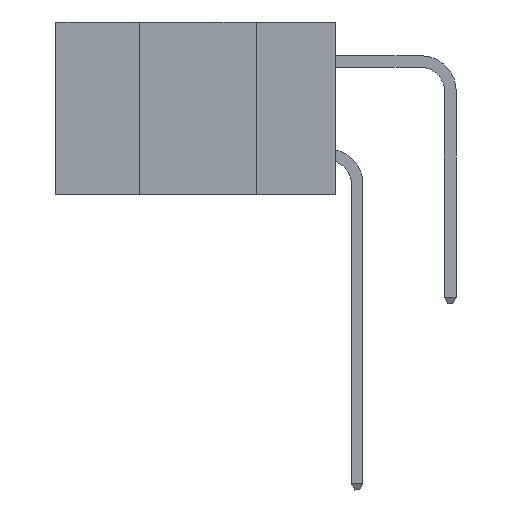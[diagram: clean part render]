
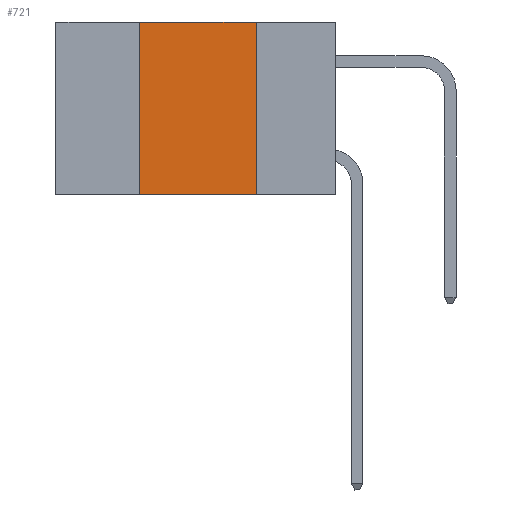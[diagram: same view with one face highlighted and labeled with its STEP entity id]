
A CAD part, left-side view. The second image highlights one B-rep face of the part: STEP entity #721.
In plain terms, the highlighted planar face has unit normal (-1, 0, 0).
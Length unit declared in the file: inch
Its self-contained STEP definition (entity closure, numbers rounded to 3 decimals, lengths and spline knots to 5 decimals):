
#721 = ADVANCED_FACE ( 'NONE', ( #14930 ), #4106, .F. ) ;
#874 = VECTOR ( 'NONE', #14177, 39.37008 ) ;
#1025 = CARTESIAN_POINT ( 'NONE',  ( 0., 0.17, -0.37 ) ) ;
#1962 = LINE ( 'NONE', #6880, #12260 ) ;
#2498 = CARTESIAN_POINT ( 'NONE',  ( 0., 0.17, 0. ) ) ;
#3488 = VERTEX_POINT ( 'NONE', #18667 ) ;
#4106 = PLANE ( 'NONE',  #18588 ) ;
#4195 = EDGE_CURVE ( 'NONE', #14457, #9766, #1962, .T. ) ;
#4528 = EDGE_CURVE ( 'NONE', #9766, #10162, #11258, .T. ) ;
#5995 = LINE ( 'NONE', #12245, #874 ) ;
#6447 = CARTESIAN_POINT ( 'NONE',  ( 0., 0.17, 0. ) ) ;
#6880 = CARTESIAN_POINT ( 'NONE',  ( 0., 0.6, 0. ) ) ;
#7224 = CARTESIAN_POINT ( 'NONE',  ( 0., 0.42, 0. ) ) ;
#7360 = VECTOR ( 'NONE', #12903, 39.37008 ) ;
#8163 = EDGE_LOOP ( 'NONE', ( #10085, #14178, #18009, #17620 ) ) ;
#8795 = CARTESIAN_POINT ( 'NONE',  ( 0., 0.6, 0. ) ) ;
#9461 = EDGE_CURVE ( 'NONE', #3488, #10162, #5995, .T. ) ;
#9766 = VERTEX_POINT ( 'NONE', #2498 ) ;
#10085 = ORIENTED_EDGE ( 'NONE', *, *, #4528, .F. ) ;
#10112 = VECTOR ( 'NONE', #10386, 39.37008 ) ;
#10149 = DIRECTION ( 'NONE',  ( 1., 0., 0. ) ) ;
#10162 = VERTEX_POINT ( 'NONE', #1025 ) ;
#10386 = DIRECTION ( 'NONE',  ( 0., 0., 1. ) ) ;
#11258 = LINE ( 'NONE', #6447, #7360 ) ;
#11547 = CARTESIAN_POINT ( 'NONE',  ( 0., 0.42, 0. ) ) ;
#11980 = EDGE_CURVE ( 'NONE', #3488, #14457, #15076, .T. ) ;
#12245 = CARTESIAN_POINT ( 'NONE',  ( 0., 0.6, -0.37 ) ) ;
#12260 = VECTOR ( 'NONE', #13120, 39.37008 ) ;
#12903 = DIRECTION ( 'NONE',  ( 0., 0., -1. ) ) ;
#13120 = DIRECTION ( 'NONE',  ( 0., -1., 0. ) ) ;
#13216 = DIRECTION ( 'NONE',  ( 0., 0., -1. ) ) ;
#14177 = DIRECTION ( 'NONE',  ( 0., -1., 0. ) ) ;
#14178 = ORIENTED_EDGE ( 'NONE', *, *, #4195, .F. ) ;
#14457 = VERTEX_POINT ( 'NONE', #11547 ) ;
#14930 = FACE_OUTER_BOUND ( 'NONE', #8163, .T. ) ;
#15076 = LINE ( 'NONE', #7224, #10112 ) ;
#17620 = ORIENTED_EDGE ( 'NONE', *, *, #9461, .T. ) ;
#18009 = ORIENTED_EDGE ( 'NONE', *, *, #11980, .F. ) ;
#18588 = AXIS2_PLACEMENT_3D ( 'NONE', #8795, #10149, #13216 ) ;
#18667 = CARTESIAN_POINT ( 'NONE',  ( 0., 0.42, -0.37 ) ) ;
